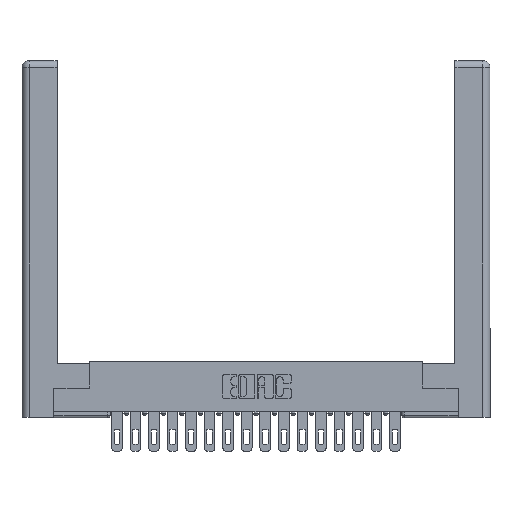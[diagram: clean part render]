
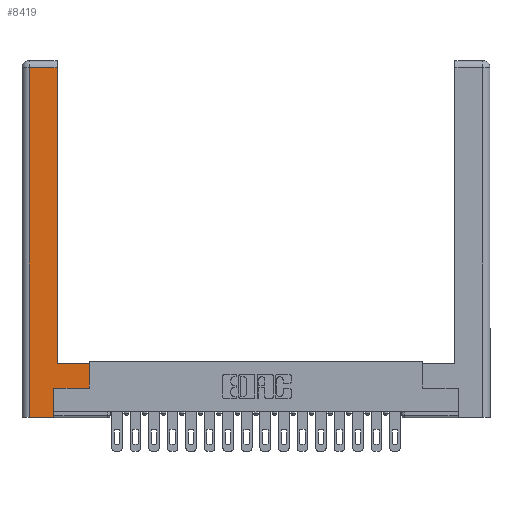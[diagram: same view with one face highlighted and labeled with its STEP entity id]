
A CAD part, top view. The second image highlights one B-rep face of the part: STEP entity #8419.
In plain terms, the highlighted planar face has unit normal (0, 0, 1).
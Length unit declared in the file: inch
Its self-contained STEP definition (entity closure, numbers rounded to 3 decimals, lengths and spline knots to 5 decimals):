
#499 = CARTESIAN_POINT ( 'NONE',  ( 0.295, 3., 0. ) ) ;
#886 = VECTOR ( 'NONE', #13115, 39.37008 ) ;
#1329 = LINE ( 'NONE', #7375, #17395 ) ;
#1558 = VECTOR ( 'NONE', #13704, 39.37008 ) ;
#1882 = PLANE ( 'NONE',  #6950 ) ;
#1888 = LINE ( 'NONE', #499, #10466 ) ;
#1983 = DIRECTION ( 'NONE',  ( -1., 0., 0. ) ) ;
#2208 = VERTEX_POINT ( 'NONE', #14726 ) ;
#2313 = VECTOR ( 'NONE', #2618, 39.37008 ) ;
#2618 = DIRECTION ( 'NONE',  ( 0., -1., 0. ) ) ;
#2952 = VERTEX_POINT ( 'NONE', #5223 ) ;
#3232 = ORIENTED_EDGE ( 'NONE', *, *, #18875, .T. ) ;
#3296 = ORIENTED_EDGE ( 'NONE', *, *, #4211, .T. ) ;
#4211 = EDGE_CURVE ( 'NONE', #6415, #18588, #1329, .T. ) ;
#4946 = EDGE_CURVE ( 'NONE', #18588, #17047, #1888, .T. ) ;
#4999 = VERTEX_POINT ( 'NONE', #14126 ) ;
#5143 = CARTESIAN_POINT ( 'NONE',  ( 0.265, 0., 0. ) ) ;
#5223 = CARTESIAN_POINT ( 'NONE',  ( 0.0615, 2.94, 0. ) ) ;
#5454 = CARTESIAN_POINT ( 'NONE',  ( 0.565, 0.45, 0. ) ) ;
#5807 = CARTESIAN_POINT ( 'NONE',  ( 0.565, 0.245, 0. ) ) ;
#5869 = ORIENTED_EDGE ( 'NONE', *, *, #15351, .T. ) ;
#5877 = ORIENTED_EDGE ( 'NONE', *, *, #19205, .T. ) ;
#6415 = VERTEX_POINT ( 'NONE', #5454 ) ;
#6923 = EDGE_CURVE ( 'NONE', #7393, #6415, #8585, .T. ) ;
#6950 = AXIS2_PLACEMENT_3D ( 'NONE', #10781, #12369, #1983 ) ;
#7375 = CARTESIAN_POINT ( 'NONE',  ( 0.295, 0.45, 0. ) ) ;
#7393 = VERTEX_POINT ( 'NONE', #5807 ) ;
#7945 = EDGE_CURVE ( 'NONE', #2208, #15025, #19345, .T. ) ;
#8419 = ADVANCED_FACE ( 'NONE', ( #9290 ), #1882, .F. ) ;
#8585 = LINE ( 'NONE', #14601, #886 ) ;
#8782 = LINE ( 'NONE', #9159, #1558 ) ;
#9155 = ORIENTED_EDGE ( 'NONE', *, *, #7945, .T. ) ;
#9159 = CARTESIAN_POINT ( 'NONE',  ( 0.0615, 2.94, 0. ) ) ;
#9290 = FACE_OUTER_BOUND ( 'NONE', #16001, .T. ) ;
#9450 = VECTOR ( 'NONE', #18785, 39.37008 ) ;
#9998 = EDGE_CURVE ( 'NONE', #15025, #7393, #13447, .T. ) ;
#10225 = CARTESIAN_POINT ( 'NONE',  ( 0.0615, 0., 0. ) ) ;
#10466 = VECTOR ( 'NONE', #13931, 39.37008 ) ;
#10781 = CARTESIAN_POINT ( 'NONE',  ( 0., 0., 0. ) ) ;
#11982 = ORIENTED_EDGE ( 'NONE', *, *, #4946, .T. ) ;
#12267 = CARTESIAN_POINT ( 'NONE',  ( 0.295, 2.94, 0. ) ) ;
#12277 = VECTOR ( 'NONE', #19490, 39.37008 ) ;
#12369 = DIRECTION ( 'NONE',  ( 0., 0., -1. ) ) ;
#13084 = DIRECTION ( 'NONE',  ( -1., 0., 0. ) ) ;
#13115 = DIRECTION ( 'NONE',  ( 0., 1., 0. ) ) ;
#13286 = ORIENTED_EDGE ( 'NONE', *, *, #9998, .T. ) ;
#13447 = LINE ( 'NONE', #19105, #12277 ) ;
#13704 = DIRECTION ( 'NONE',  ( -1., 0., 0. ) ) ;
#13931 = DIRECTION ( 'NONE',  ( 0., 1., 0. ) ) ;
#14023 = LINE ( 'NONE', #5143, #9450 ) ;
#14126 = CARTESIAN_POINT ( 'NONE',  ( 0.0615, 0., 0. ) ) ;
#14162 = CARTESIAN_POINT ( 'NONE',  ( 0.295, 0.45, 0. ) ) ;
#14601 = CARTESIAN_POINT ( 'NONE',  ( 0.565, 0.45, 0. ) ) ;
#14726 = CARTESIAN_POINT ( 'NONE',  ( 0.265, 0., 0. ) ) ;
#15025 = VERTEX_POINT ( 'NONE', #16377 ) ;
#15351 = EDGE_CURVE ( 'NONE', #2952, #4999, #17760, .T. ) ;
#16001 = EDGE_LOOP ( 'NONE', ( #11982, #5877, #5869, #3232, #9155, #13286, #18646, #3296 ) ) ;
#16377 = CARTESIAN_POINT ( 'NONE',  ( 0.265, 0.245, 0. ) ) ;
#17008 = VECTOR ( 'NONE', #17960, 39.37008 ) ;
#17047 = VERTEX_POINT ( 'NONE', #12267 ) ;
#17395 = VECTOR ( 'NONE', #13084, 39.37008 ) ;
#17760 = LINE ( 'NONE', #10225, #2313 ) ;
#17871 = CARTESIAN_POINT ( 'NONE',  ( 0.265, 0.245, 0. ) ) ;
#17960 = DIRECTION ( 'NONE',  ( 0., 1., 0. ) ) ;
#18588 = VERTEX_POINT ( 'NONE', #14162 ) ;
#18646 = ORIENTED_EDGE ( 'NONE', *, *, #6923, .T. ) ;
#18785 = DIRECTION ( 'NONE',  ( 1., 0., 0. ) ) ;
#18875 = EDGE_CURVE ( 'NONE', #4999, #2208, #14023, .T. ) ;
#19105 = CARTESIAN_POINT ( 'NONE',  ( 0.565, 0.245, 0. ) ) ;
#19205 = EDGE_CURVE ( 'NONE', #17047, #2952, #8782, .T. ) ;
#19345 = LINE ( 'NONE', #17871, #17008 ) ;
#19490 = DIRECTION ( 'NONE',  ( 1., 0., 0. ) ) ;
